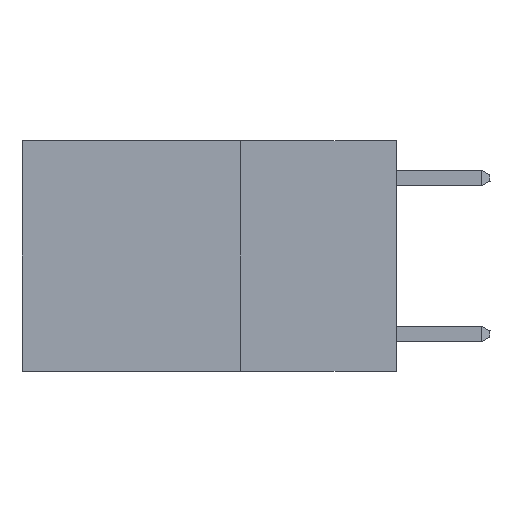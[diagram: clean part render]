
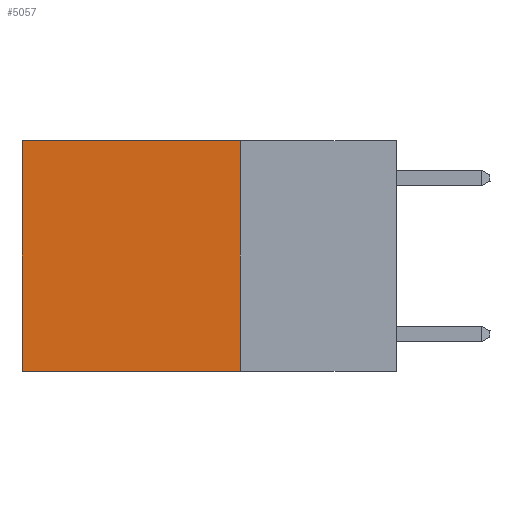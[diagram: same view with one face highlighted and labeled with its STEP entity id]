
A CAD part, left-side view. The second image highlights one B-rep face of the part: STEP entity #5057.
In plain terms, the highlighted planar face has unit normal (-1, 0, 0).
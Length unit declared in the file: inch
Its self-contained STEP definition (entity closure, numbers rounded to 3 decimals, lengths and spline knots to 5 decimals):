
#106 = DIRECTION ( 'NONE',  ( 0., 0., -1. ) ) ;
#175 = CARTESIAN_POINT ( 'NONE',  ( 0.2625, 0.25, 0. ) ) ;
#213 = VERTEX_POINT ( 'NONE', #7196 ) ;
#297 = CARTESIAN_POINT ( 'NONE',  ( 0.2625, 0.25, -0.37 ) ) ;
#500 = ORIENTED_EDGE ( 'NONE', *, *, #7901, .T. ) ;
#652 = CARTESIAN_POINT ( 'NONE',  ( 0.2625, 0.6, 0. ) ) ;
#657 = ORIENTED_EDGE ( 'NONE', *, *, #9602, .F. ) ;
#694 = ORIENTED_EDGE ( 'NONE', *, *, #731, .T. ) ;
#731 = EDGE_CURVE ( 'NONE', #3192, #213, #11108, .T. ) ;
#802 = EDGE_LOOP ( 'NONE', ( #500, #657, #2204, #694 ) ) ;
#1061 = VECTOR ( 'NONE', #9525, 39.37008 ) ;
#2131 = LINE ( 'NONE', #7408, #6657 ) ;
#2166 = AXIS2_PLACEMENT_3D ( 'NONE', #175, #5364, #106 ) ;
#2204 = ORIENTED_EDGE ( 'NONE', *, *, #3317, .F. ) ;
#3192 = VERTEX_POINT ( 'NONE', #7650 ) ;
#3252 = DIRECTION ( 'NONE',  ( 0., 1., 0. ) ) ;
#3317 = EDGE_CURVE ( 'NONE', #3192, #8754, #10975, .T. ) ;
#3410 = VERTEX_POINT ( 'NONE', #4271 ) ;
#4067 = VECTOR ( 'NONE', #3252, 39.37008 ) ;
#4271 = CARTESIAN_POINT ( 'NONE',  ( 0.2625, 0.6, -0.37 ) ) ;
#4691 = DIRECTION ( 'NONE',  ( 0., 1., 0. ) ) ;
#4740 = CARTESIAN_POINT ( 'NONE',  ( 0.2625, 0.25, 0. ) ) ;
#5057 = ADVANCED_FACE ( 'NONE', ( #8423 ), #5402, .F. ) ;
#5188 = VECTOR ( 'NONE', #5709, 39.37008 ) ;
#5364 = DIRECTION ( 'NONE',  ( 1., 0., 0. ) ) ;
#5402 = PLANE ( 'NONE',  #2166 ) ;
#5709 = DIRECTION ( 'NONE',  ( 0., 0., -1. ) ) ;
#6657 = VECTOR ( 'NONE', #4691, 39.37008 ) ;
#6751 = CARTESIAN_POINT ( 'NONE',  ( 0.2625, 0.25, 0. ) ) ;
#7196 = CARTESIAN_POINT ( 'NONE',  ( 0.2625, 0.6, 0. ) ) ;
#7408 = CARTESIAN_POINT ( 'NONE',  ( 0.2625, 0.25, -0.37 ) ) ;
#7650 = CARTESIAN_POINT ( 'NONE',  ( 0.2625, 0.25, 0. ) ) ;
#7901 = EDGE_CURVE ( 'NONE', #213, #3410, #10822, .T. ) ;
#8423 = FACE_OUTER_BOUND ( 'NONE', #802, .T. ) ;
#8754 = VERTEX_POINT ( 'NONE', #297 ) ;
#9525 = DIRECTION ( 'NONE',  ( 0., 0., -1. ) ) ;
#9602 = EDGE_CURVE ( 'NONE', #8754, #3410, #2131, .T. ) ;
#10822 = LINE ( 'NONE', #652, #1061 ) ;
#10975 = LINE ( 'NONE', #4740, #5188 ) ;
#11108 = LINE ( 'NONE', #6751, #4067 ) ;
